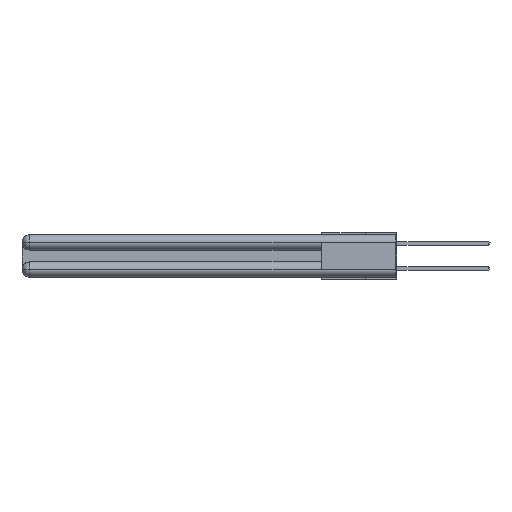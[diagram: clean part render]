
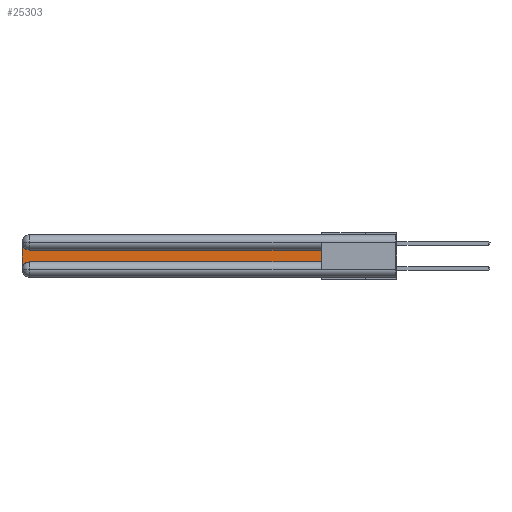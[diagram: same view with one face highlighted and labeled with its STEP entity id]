
A CAD part, left-side view. The second image highlights one B-rep face of the part: STEP entity #25303.
In plain terms, the highlighted planar face has unit normal (-1, 0, 0).
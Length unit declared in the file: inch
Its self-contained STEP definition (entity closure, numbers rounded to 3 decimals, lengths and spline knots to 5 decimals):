
#110 = EDGE_CURVE ( 'NONE', #6043, #13605, #20753, .T. ) ;
#1019 = CIRCLE ( 'NONE', #22133, 0.06 ) ;
#1207 = CARTESIAN_POINT ( 'NONE',  ( 0.075, 3., -0.2775 ) ) ;
#1901 = EDGE_CURVE ( 'NONE', #22010, #17417, #1019, .T. ) ;
#2177 = CARTESIAN_POINT ( 'NONE',  ( 0.075, 3., -0.2175 ) ) ;
#3187 = DIRECTION ( 'NONE',  ( 0., 0., -1. ) ) ;
#3474 = CARTESIAN_POINT ( 'NONE',  ( 0.075, 0.6, -0.1225 ) ) ;
#4047 = PLANE ( 'NONE',  #24906 ) ;
#4506 = CARTESIAN_POINT ( 'NONE',  ( 0.075, 0.6, -0.2175 ) ) ;
#4853 = LINE ( 'NONE', #3474, #21573 ) ;
#5201 = CARTESIAN_POINT ( 'NONE',  ( 0.075, 2.94, -0.2175 ) ) ;
#5706 = ORIENTED_EDGE ( 'NONE', *, *, #12261, .T. ) ;
#5763 = DIRECTION ( 'NONE',  ( 0., 0., -1. ) ) ;
#6043 = VERTEX_POINT ( 'NONE', #18217 ) ;
#6173 = CARTESIAN_POINT ( 'NONE',  ( 0.075, 2.94, -0.0625 ) ) ;
#6424 = CARTESIAN_POINT ( 'NONE',  ( 0.075, 3., -0.1225 ) ) ;
#6801 = DIRECTION ( 'NONE',  ( 0., 0., -1. ) ) ;
#8742 = DIRECTION ( 'NONE',  ( 0., 0., -1. ) ) ;
#8819 = EDGE_CURVE ( 'NONE', #10099, #20491, #25042, .T. ) ;
#10099 = VERTEX_POINT ( 'NONE', #23113 ) ;
#10208 = CARTESIAN_POINT ( 'NONE',  ( 0.075, 0.6, -0.1225 ) ) ;
#10493 = DIRECTION ( 'NONE',  ( 0., 1., 0. ) ) ;
#11326 = LINE ( 'NONE', #2177, #23668 ) ;
#12261 = EDGE_CURVE ( 'NONE', #20491, #6043, #4853, .T. ) ;
#13605 = VERTEX_POINT ( 'NONE', #20014 ) ;
#15024 = CARTESIAN_POINT ( 'NONE',  ( 0.075, 2.94, -0.2775 ) ) ;
#15784 = FACE_OUTER_BOUND ( 'NONE', #29550, .T. ) ;
#16924 = ORIENTED_EDGE ( 'NONE', *, *, #24532, .T. ) ;
#17176 = CARTESIAN_POINT ( 'NONE',  ( 0.075, 0.6, -0.2175 ) ) ;
#17417 = VERTEX_POINT ( 'NONE', #5201 ) ;
#18217 = CARTESIAN_POINT ( 'NONE',  ( 0.075, 2.94, -0.1225 ) ) ;
#19608 = DIRECTION ( 'NONE',  ( 0., 0., 1. ) ) ;
#19670 = EDGE_CURVE ( 'NONE', #13605, #22010, #11326, .T. ) ;
#19948 = DIRECTION ( 'NONE',  ( 1., 0., 0. ) ) ;
#20014 = CARTESIAN_POINT ( 'NONE',  ( 0.075, 3., -0.0625 ) ) ;
#20491 = VERTEX_POINT ( 'NONE', #10208 ) ;
#20753 = CIRCLE ( 'NONE', #25177, 0.06 ) ;
#21573 = VECTOR ( 'NONE', #10493, 39.37008 ) ;
#22010 = VERTEX_POINT ( 'NONE', #1207 ) ;
#22133 = AXIS2_PLACEMENT_3D ( 'NONE', #15024, #28585, #3187 ) ;
#22611 = DIRECTION ( 'NONE',  ( 1., 0., 0. ) ) ;
#23113 = CARTESIAN_POINT ( 'NONE',  ( 0.075, 0.6, -0.2175 ) ) ;
#23581 = VECTOR ( 'NONE', #19608, 39.37008 ) ;
#23668 = VECTOR ( 'NONE', #6801, 39.37008 ) ;
#24049 = ORIENTED_EDGE ( 'NONE', *, *, #8819, .T. ) ;
#24532 = EDGE_CURVE ( 'NONE', #17417, #10099, #29227, .T. ) ;
#24906 = AXIS2_PLACEMENT_3D ( 'NONE', #6424, #22611, #8742 ) ;
#25042 = LINE ( 'NONE', #17176, #23581 ) ;
#25177 = AXIS2_PLACEMENT_3D ( 'NONE', #6173, #19948, #5763 ) ;
#25264 = ORIENTED_EDGE ( 'NONE', *, *, #19670, .T. ) ;
#25303 = ADVANCED_FACE ( 'NONE', ( #15784 ), #4047, .F. ) ;
#26324 = VECTOR ( 'NONE', #27559, 39.37008 ) ;
#27559 = DIRECTION ( 'NONE',  ( 0., -1., 0. ) ) ;
#27922 = ORIENTED_EDGE ( 'NONE', *, *, #1901, .T. ) ;
#28585 = DIRECTION ( 'NONE',  ( 1., 0., 0. ) ) ;
#29227 = LINE ( 'NONE', #4506, #26324 ) ;
#29550 = EDGE_LOOP ( 'NONE', ( #5706, #29865, #25264, #27922, #16924, #24049 ) ) ;
#29865 = ORIENTED_EDGE ( 'NONE', *, *, #110, .T. ) ;
